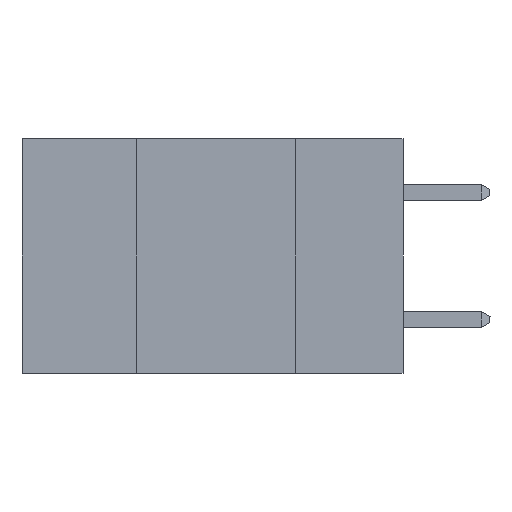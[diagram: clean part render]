
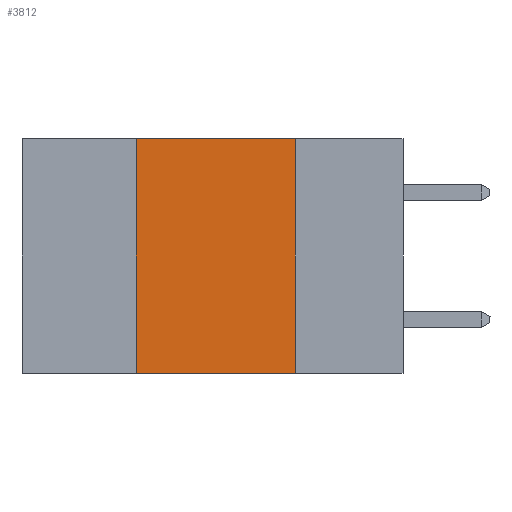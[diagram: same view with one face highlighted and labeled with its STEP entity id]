
A CAD part, left-side view. The second image highlights one B-rep face of the part: STEP entity #3812.
In plain terms, the highlighted planar face has unit normal (-1, 0, 0).
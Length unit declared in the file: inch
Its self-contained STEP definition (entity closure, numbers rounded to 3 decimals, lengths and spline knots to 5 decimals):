
#2403 = VERTEX_POINT ( 'NONE', #28770 ) ;
#3381 = EDGE_CURVE ( 'NONE', #34622, #2403, #43606, .T. ) ;
#3812 = ADVANCED_FACE ( 'NONE', ( #7454 ), #46673, .F. ) ;
#7454 = FACE_OUTER_BOUND ( 'NONE', #16510, .T. ) ;
#8026 = VECTOR ( 'NONE', #16643, 39.37008 ) ;
#8615 = VERTEX_POINT ( 'NONE', #10326 ) ;
#10218 = EDGE_CURVE ( 'NONE', #2403, #8615, #28965, .T. ) ;
#10326 = CARTESIAN_POINT ( 'NONE',  ( 0., 0.17, -0.37 ) ) ;
#12662 = VECTOR ( 'NONE', #13678, 39.37008 ) ;
#13678 = DIRECTION ( 'NONE',  ( 0., -1., 0. ) ) ;
#14972 = VERTEX_POINT ( 'NONE', #15801 ) ;
#15801 = CARTESIAN_POINT ( 'NONE',  ( 0., 0.42, -0.37 ) ) ;
#16205 = ORIENTED_EDGE ( 'NONE', *, *, #3381, .F. ) ;
#16510 = EDGE_LOOP ( 'NONE', ( #26667, #16205, #24146, #38817 ) ) ;
#16643 = DIRECTION ( 'NONE',  ( 0., 0., 1. ) ) ;
#17554 = AXIS2_PLACEMENT_3D ( 'NONE', #46437, #28726, #32535 ) ;
#17566 = CARTESIAN_POINT ( 'NONE',  ( 0., 0.6, 0. ) ) ;
#23677 = VECTOR ( 'NONE', #32128, 39.37008 ) ;
#24146 = ORIENTED_EDGE ( 'NONE', *, *, #36381, .F. ) ;
#24301 = LINE ( 'NONE', #27170, #8026 ) ;
#26667 = ORIENTED_EDGE ( 'NONE', *, *, #10218, .F. ) ;
#27170 = CARTESIAN_POINT ( 'NONE',  ( 0., 0.42, 0. ) ) ;
#28726 = DIRECTION ( 'NONE',  ( 1., 0., 0. ) ) ;
#28770 = CARTESIAN_POINT ( 'NONE',  ( 0., 0.17, 0. ) ) ;
#28965 = LINE ( 'NONE', #39738, #31694 ) ;
#31513 = CARTESIAN_POINT ( 'NONE',  ( 0., 0.42, 0. ) ) ;
#31694 = VECTOR ( 'NONE', #37092, 39.37008 ) ;
#32128 = DIRECTION ( 'NONE',  ( 0., -1., 0. ) ) ;
#32535 = DIRECTION ( 'NONE',  ( 0., 0., -1. ) ) ;
#34622 = VERTEX_POINT ( 'NONE', #31513 ) ;
#36381 = EDGE_CURVE ( 'NONE', #14972, #34622, #24301, .T. ) ;
#36984 = EDGE_CURVE ( 'NONE', #14972, #8615, #42849, .T. ) ;
#37092 = DIRECTION ( 'NONE',  ( 0., 0., -1. ) ) ;
#38817 = ORIENTED_EDGE ( 'NONE', *, *, #36984, .T. ) ;
#39738 = CARTESIAN_POINT ( 'NONE',  ( 0., 0.17, 0. ) ) ;
#42849 = LINE ( 'NONE', #46439, #12662 ) ;
#43606 = LINE ( 'NONE', #17566, #23677 ) ;
#46437 = CARTESIAN_POINT ( 'NONE',  ( 0., 0.6, 0. ) ) ;
#46439 = CARTESIAN_POINT ( 'NONE',  ( 0., 0.6, -0.37 ) ) ;
#46673 = PLANE ( 'NONE',  #17554 ) ;
